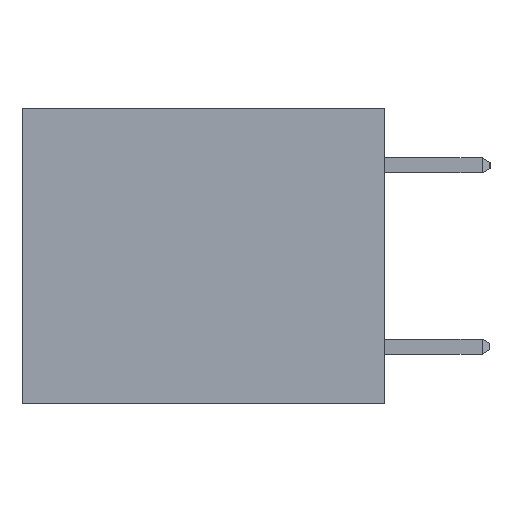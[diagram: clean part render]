
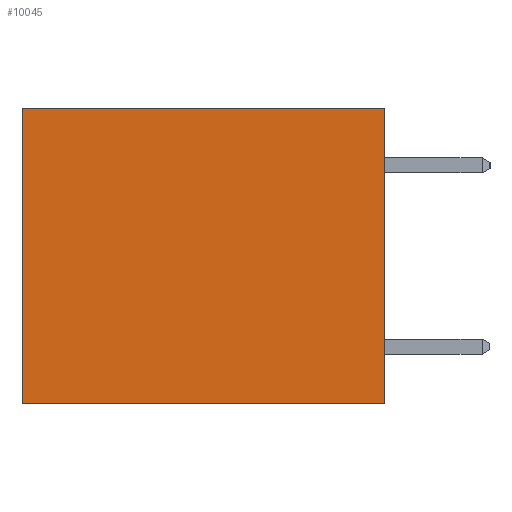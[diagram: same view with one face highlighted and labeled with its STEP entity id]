
A CAD part, left-side view. The second image highlights one B-rep face of the part: STEP entity #10045.
In plain terms, the highlighted planar face has unit normal (-1, 0, 0).
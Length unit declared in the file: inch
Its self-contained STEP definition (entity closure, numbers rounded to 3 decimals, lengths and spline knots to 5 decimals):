
#164 = VECTOR ( 'NONE', #12670, 39.37008 ) ;
#454 = CARTESIAN_POINT ( 'NONE',  ( 0.3165, 0., 0. ) ) ;
#2752 = ORIENTED_EDGE ( 'NONE', *, *, #6817, .T. ) ;
#2862 = CARTESIAN_POINT ( 'NONE',  ( 0.3165, 0.6, -0.49 ) ) ;
#2896 = CARTESIAN_POINT ( 'NONE',  ( 0.3165, 0.6, -0.49 ) ) ;
#4164 = LINE ( 'NONE', #454, #164 ) ;
#4176 = LINE ( 'NONE', #8463, #9073 ) ;
#4363 = LINE ( 'NONE', #14396, #6107 ) ;
#4542 = LINE ( 'NONE', #2896, #13627 ) ;
#5834 = VERTEX_POINT ( 'NONE', #14170 ) ;
#6107 = VECTOR ( 'NONE', #8051, 39.37008 ) ;
#6420 = EDGE_CURVE ( 'NONE', #9904, #6566, #4176, .T. ) ;
#6566 = VERTEX_POINT ( 'NONE', #9769 ) ;
#6817 = EDGE_CURVE ( 'NONE', #9904, #5834, #4164, .T. ) ;
#7637 = ORIENTED_EDGE ( 'NONE', *, *, #14387, .T. ) ;
#7821 = DIRECTION ( 'NONE',  ( 1., 0., 0. ) ) ;
#8051 = DIRECTION ( 'NONE',  ( 0., 1., 0. ) ) ;
#8463 = CARTESIAN_POINT ( 'NONE',  ( 0.3165, 0., -0.49 ) ) ;
#8498 = EDGE_LOOP ( 'NONE', ( #7637, #12930, #9302, #2752 ) ) ;
#9073 = VECTOR ( 'NONE', #14150, 39.37008 ) ;
#9302 = ORIENTED_EDGE ( 'NONE', *, *, #6420, .F. ) ;
#9769 = CARTESIAN_POINT ( 'NONE',  ( 0.3165, 0., -0.49 ) ) ;
#9904 = VERTEX_POINT ( 'NONE', #12054 ) ;
#10045 = ADVANCED_FACE ( 'NONE', ( #13964 ), #13378, .F. ) ;
#10072 = DIRECTION ( 'NONE',  ( 0., 0., -1. ) ) ;
#10122 = CARTESIAN_POINT ( 'NONE',  ( 0.3165, 0., -0.49 ) ) ;
#10290 = EDGE_CURVE ( 'NONE', #6566, #12070, #4363, .T. ) ;
#12054 = CARTESIAN_POINT ( 'NONE',  ( 0.3165, 0., 0. ) ) ;
#12070 = VERTEX_POINT ( 'NONE', #2862 ) ;
#12670 = DIRECTION ( 'NONE',  ( 0., 1., 0. ) ) ;
#12930 = ORIENTED_EDGE ( 'NONE', *, *, #10290, .F. ) ;
#12989 = DIRECTION ( 'NONE',  ( 0., 0., -1. ) ) ;
#13378 = PLANE ( 'NONE',  #13854 ) ;
#13627 = VECTOR ( 'NONE', #12989, 39.37008 ) ;
#13854 = AXIS2_PLACEMENT_3D ( 'NONE', #10122, #7821, #10072 ) ;
#13964 = FACE_OUTER_BOUND ( 'NONE', #8498, .T. ) ;
#14150 = DIRECTION ( 'NONE',  ( 0., 0., -1. ) ) ;
#14170 = CARTESIAN_POINT ( 'NONE',  ( 0.3165, 0.6, 0. ) ) ;
#14387 = EDGE_CURVE ( 'NONE', #5834, #12070, #4542, .T. ) ;
#14396 = CARTESIAN_POINT ( 'NONE',  ( 0.3165, 0., -0.49 ) ) ;
